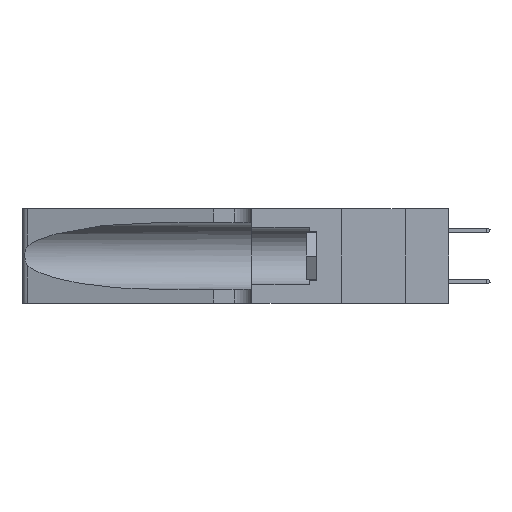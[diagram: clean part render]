
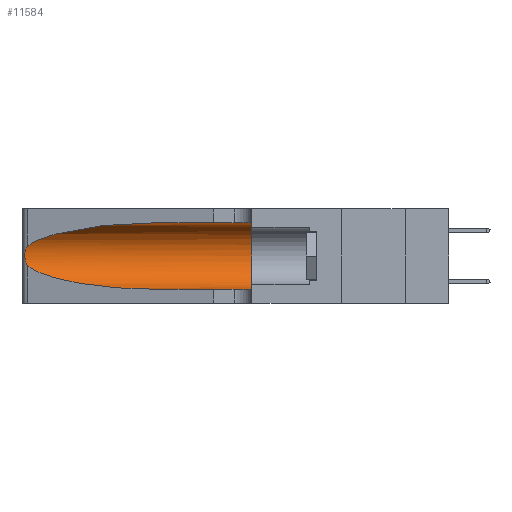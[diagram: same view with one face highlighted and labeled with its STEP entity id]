
A CAD part, left-side view. The second image highlights one B-rep face of the part: STEP entity #11584.
In plain terms, the highlighted cylindrical face has radius 3.308 mm (diameter 6.617 mm), a partial arc.
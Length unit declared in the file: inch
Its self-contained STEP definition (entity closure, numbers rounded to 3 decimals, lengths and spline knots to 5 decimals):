
#174 = ORIENTED_EDGE ( 'NONE', *, *, #19427, .F. ) ;
#311 = B_SPLINE_CURVE_WITH_KNOTS ( 'NONE', 3,
 ( #33329, #12569, #15184, #1880, #20447, #4637, #23032, #7400, #25641, #10082, #28208, #12684, #30813, #15298 ),
 .UNSPECIFIED., .F., .F.,
 ( 4, 2, 2, 2, 2, 2, 4 ),
 ( 0., 0.00027, 0.00053, 0.00107, 0.0016, 0.00187, 0.00214 ),
 .UNSPECIFIED. ) ;
#1277 = CARTESIAN_POINT ( 'NONE',  ( 0.1305, 0.72297, 0.05475 ) ) ;
#1880 = CARTESIAN_POINT ( 'NONE',  ( 0.25787, 1.23484, 0.2124 ) ) ;
#2647 = EDGE_CURVE ( 'NONE', #11658, #25872, #311, .T. ) ;
#3212 = CARTESIAN_POINT ( 'NONE',  ( 0.1305, 1.61858, 0.05475 ) ) ;
#3819 = CARTESIAN_POINT ( 'NONE',  ( 0.25487, 1.22718, 0.14631 ) ) ;
#4148 = VECTOR ( 'NONE', #31969, 39.37008 ) ;
#4438 = VERTEX_POINT ( 'NONE', #13152 ) ;
#4637 = CARTESIAN_POINT ( 'NONE',  ( 0.26018, 1.23835, 0.19895 ) ) ;
#4996 = LINE ( 'NONE', #3212, #4148 ) ;
#5293 = CARTESIAN_POINT ( 'NONE',  ( 0.1305, 1.61858, 0.185 ) ) ;
#6132 = ORIENTED_EDGE ( 'NONE', *, *, #2647, .T. ) ;
#7069 = FACE_OUTER_BOUND ( 'NONE', #16871, .T. ) ;
#7259 = CARTESIAN_POINT ( 'NONE',  ( 0.1305, 0.72297, 0.31525 ) ) ;
#7400 = CARTESIAN_POINT ( 'NONE',  ( 0.26075, 1.23896, 0.178 ) ) ;
#7503 = CARTESIAN_POINT ( 'NONE',  ( 0.1305, 0.72297, 0.31525 ) ) ;
#7568 = EDGE_CURVE ( 'NONE', #17393, #9508, #27207, .T. ) ;
#8269 = CARTESIAN_POINT ( 'NONE',  ( 0.25487, 1.22718, 0.22369 ) ) ;
#8489 = ORIENTED_EDGE ( 'NONE', *, *, #29425, .T. ) ;
#9141 = AXIS2_PLACEMENT_3D ( 'NONE', #5293, #10690, #13282 ) ;
#9508 = VERTEX_POINT ( 'NONE', #30634 ) ;
#9636 = DIRECTION ( 'NONE',  ( 0., -1., 0. ) ) ;
#10082 = CARTESIAN_POINT ( 'NONE',  ( 0.25856, 1.23593, 0.16098 ) ) ;
#10179 = CARTESIAN_POINT ( 'NONE',  ( 0.2373, 1.15595, 0.28018 ) ) ;
#10319 =( BOUNDED_CURVE ( )  B_SPLINE_CURVE ( 3, ( #7503, #20547, #10179, #28316 ),
 .UNSPECIFIED., .F., .T. ) 
 B_SPLINE_CURVE_WITH_KNOTS ( ( 4, 4 ),
 ( 1.5708, 2.84003 ),
 .UNSPECIFIED. ) 
 CURVE ( )  GEOMETRIC_REPRESENTATION_ITEM ( )  RATIONAL_B_SPLINE_CURVE ( ( 1., 0.87, 0.87, 1. ) ) 
 REPRESENTATION_ITEM ( '' )  );
#10690 = DIRECTION ( 'NONE',  ( 0., -1., 0. ) ) ;
#11397 = ORIENTED_EDGE ( 'NONE', *, *, #14144, .T. ) ;
#11584 = ADVANCED_FACE ( 'NONE', ( #7069 ), #33923, .F. ) ;
#11658 = VERTEX_POINT ( 'NONE', #8269 ) ;
#12569 = CARTESIAN_POINT ( 'NONE',  ( 0.25555, 1.22994, 0.2215 ) ) ;
#12684 = CARTESIAN_POINT ( 'NONE',  ( 0.25639, 1.23186, 0.15144 ) ) ;
#13152 = CARTESIAN_POINT ( 'NONE',  ( 0.1305, 0.72297, 0.05475 ) ) ;
#13282 = DIRECTION ( 'NONE',  ( 0., 0., -1. ) ) ;
#13845 =( BOUNDED_CURVE ( )  B_SPLINE_CURVE ( 3, ( #27537, #30128, #17238, #1277 ),
 .UNSPECIFIED., .F., .F. ) 
 B_SPLINE_CURVE_WITH_KNOTS ( ( 4, 4 ),
 ( 3.44316, 4.71239 ),
 .UNSPECIFIED. ) 
 CURVE ( )  GEOMETRIC_REPRESENTATION_ITEM ( )  RATIONAL_B_SPLINE_CURVE ( ( 1., 0.87, 0.87, 1. ) ) 
 REPRESENTATION_ITEM ( '' )  );
#14144 = EDGE_CURVE ( 'NONE', #16627, #11658, #10319, .T. ) ;
#14850 = CARTESIAN_POINT ( 'NONE',  ( 0.1305, 1.61858, 0.31525 ) ) ;
#15184 = CARTESIAN_POINT ( 'NONE',  ( 0.25639, 1.23184, 0.21858 ) ) ;
#15298 = CARTESIAN_POINT ( 'NONE',  ( 0.25487, 1.22718, 0.14631 ) ) ;
#15877 = DIRECTION ( 'NONE',  ( 0., 1., 0. ) ) ;
#16627 = VERTEX_POINT ( 'NONE', #7259 ) ;
#16871 = EDGE_LOOP ( 'NONE', ( #11397, #6132, #8489, #27428, #32432, #174 ) ) ;
#17238 = CARTESIAN_POINT ( 'NONE',  ( 0.18966, 0.96281, 0.05475 ) ) ;
#17393 = VERTEX_POINT ( 'NONE', #17985 ) ;
#17985 = CARTESIAN_POINT ( 'NONE',  ( 0.1305, 0.35, 0.31525 ) ) ;
#18677 = AXIS2_PLACEMENT_3D ( 'NONE', #31393, #15877, #34001 ) ;
#19427 = EDGE_CURVE ( 'NONE', #16627, #17393, #23489, .T. ) ;
#20447 = CARTESIAN_POINT ( 'NONE',  ( 0.25854, 1.2359, 0.20912 ) ) ;
#20547 = CARTESIAN_POINT ( 'NONE',  ( 0.18966, 0.96281, 0.31525 ) ) ;
#22665 = VECTOR ( 'NONE', #9636, 39.37008 ) ;
#23032 = CARTESIAN_POINT ( 'NONE',  ( 0.26075, 1.23896, 0.19203 ) ) ;
#23489 = LINE ( 'NONE', #14850, #22665 ) ;
#25641 = CARTESIAN_POINT ( 'NONE',  ( 0.26017, 1.23833, 0.17102 ) ) ;
#25872 = VERTEX_POINT ( 'NONE', #3819 ) ;
#27207 = CIRCLE ( 'NONE', #18677, 0.13025 ) ;
#27428 = ORIENTED_EDGE ( 'NONE', *, *, #33232, .T. ) ;
#27537 = CARTESIAN_POINT ( 'NONE',  ( 0.25487, 1.22718, 0.14631 ) ) ;
#28208 = CARTESIAN_POINT ( 'NONE',  ( 0.25789, 1.23486, 0.15765 ) ) ;
#28316 = CARTESIAN_POINT ( 'NONE',  ( 0.25487, 1.22718, 0.22369 ) ) ;
#29425 = EDGE_CURVE ( 'NONE', #25872, #4438, #13845, .T. ) ;
#30128 = CARTESIAN_POINT ( 'NONE',  ( 0.2373, 1.15595, 0.08982 ) ) ;
#30634 = CARTESIAN_POINT ( 'NONE',  ( 0.1305, 0.35, 0.05475 ) ) ;
#30813 = CARTESIAN_POINT ( 'NONE',  ( 0.25555, 1.22993, 0.14849 ) ) ;
#31393 = CARTESIAN_POINT ( 'NONE',  ( 0.1305, 0.35, 0.185 ) ) ;
#31969 = DIRECTION ( 'NONE',  ( 0., -1., 0. ) ) ;
#32432 = ORIENTED_EDGE ( 'NONE', *, *, #7568, .F. ) ;
#33232 = EDGE_CURVE ( 'NONE', #4438, #9508, #4996, .T. ) ;
#33329 = CARTESIAN_POINT ( 'NONE',  ( 0.25487, 1.22718, 0.22369 ) ) ;
#33923 = CYLINDRICAL_SURFACE ( 'NONE', #9141, 0.13025 ) ;
#34001 = DIRECTION ( 'NONE',  ( 0., 0., 1. ) ) ;
